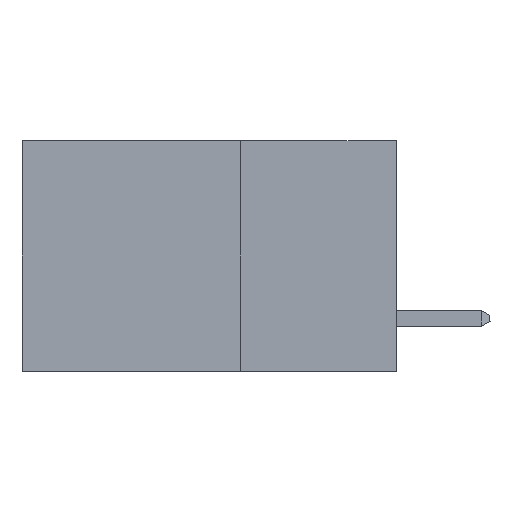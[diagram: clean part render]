
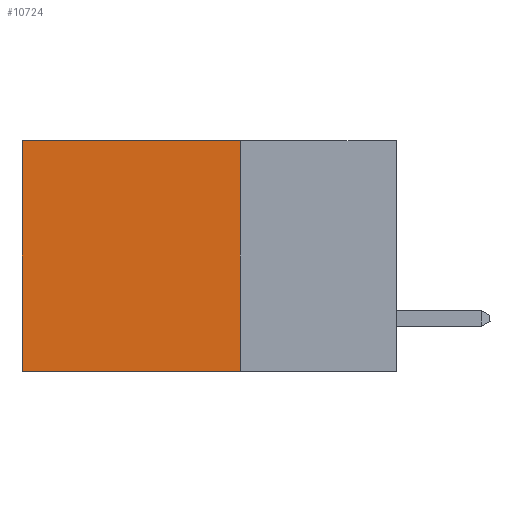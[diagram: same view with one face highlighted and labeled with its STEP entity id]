
A CAD part, left-side view. The second image highlights one B-rep face of the part: STEP entity #10724.
In plain terms, the highlighted planar face has unit normal (-1, 0, 0).
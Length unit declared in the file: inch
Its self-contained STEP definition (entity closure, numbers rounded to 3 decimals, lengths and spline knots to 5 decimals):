
#250 = DIRECTION ( 'NONE',  ( 0., 0., -1. ) ) ;
#745 = CARTESIAN_POINT ( 'NONE',  ( 0.298, 0.25, -0.37 ) ) ;
#1010 = DIRECTION ( 'NONE',  ( 0., 0., -1. ) ) ;
#1066 = DIRECTION ( 'NONE',  ( 0., 0., -1. ) ) ;
#1595 = CARTESIAN_POINT ( 'NONE',  ( 0.298, 0.6, 0. ) ) ;
#2368 = CARTESIAN_POINT ( 'NONE',  ( 0.298, 0.25, 0. ) ) ;
#3528 = VECTOR ( 'NONE', #7674, 39.37008 ) ;
#4244 = ORIENTED_EDGE ( 'NONE', *, *, #6681, .T. ) ;
#4629 = EDGE_LOOP ( 'NONE', ( #4244, #6100, #6866, #18525 ) ) ;
#4815 = VECTOR ( 'NONE', #18467, 39.37008 ) ;
#6100 = ORIENTED_EDGE ( 'NONE', *, *, #11035, .F. ) ;
#6117 = CARTESIAN_POINT ( 'NONE',  ( 0.298, 0.25, 0. ) ) ;
#6582 = EDGE_CURVE ( 'NONE', #9465, #8187, #16384, .T. ) ;
#6681 = EDGE_CURVE ( 'NONE', #8187, #18681, #7341, .T. ) ;
#6849 = VECTOR ( 'NONE', #1010, 39.37008 ) ;
#6866 = ORIENTED_EDGE ( 'NONE', *, *, #17696, .F. ) ;
#7099 = CARTESIAN_POINT ( 'NONE',  ( 0.298, 0.6, -0.37 ) ) ;
#7341 = LINE ( 'NONE', #1595, #6849 ) ;
#7674 = DIRECTION ( 'NONE',  ( 0., 1., 0. ) ) ;
#8187 = VERTEX_POINT ( 'NONE', #18129 ) ;
#9465 = VERTEX_POINT ( 'NONE', #2368 ) ;
#9950 = DIRECTION ( 'NONE',  ( 1., 0., 0. ) ) ;
#10078 = VERTEX_POINT ( 'NONE', #745 ) ;
#10724 = ADVANCED_FACE ( 'NONE', ( #15791 ), #14235, .F. ) ;
#10839 = LINE ( 'NONE', #14945, #3528 ) ;
#11035 = EDGE_CURVE ( 'NONE', #10078, #18681, #10839, .T. ) ;
#11968 = LINE ( 'NONE', #12090, #18720 ) ;
#12090 = CARTESIAN_POINT ( 'NONE',  ( 0.298, 0.25, 0. ) ) ;
#14235 = PLANE ( 'NONE',  #17893 ) ;
#14945 = CARTESIAN_POINT ( 'NONE',  ( 0.298, 0.25, -0.37 ) ) ;
#15791 = FACE_OUTER_BOUND ( 'NONE', #4629, .T. ) ;
#16384 = LINE ( 'NONE', #6117, #4815 ) ;
#17696 = EDGE_CURVE ( 'NONE', #9465, #10078, #11968, .T. ) ;
#17893 = AXIS2_PLACEMENT_3D ( 'NONE', #18586, #9950, #1066 ) ;
#18129 = CARTESIAN_POINT ( 'NONE',  ( 0.298, 0.6, 0. ) ) ;
#18467 = DIRECTION ( 'NONE',  ( 0., 1., 0. ) ) ;
#18525 = ORIENTED_EDGE ( 'NONE', *, *, #6582, .T. ) ;
#18586 = CARTESIAN_POINT ( 'NONE',  ( 0.298, 0.25, 0. ) ) ;
#18681 = VERTEX_POINT ( 'NONE', #7099 ) ;
#18720 = VECTOR ( 'NONE', #250, 39.37008 ) ;
